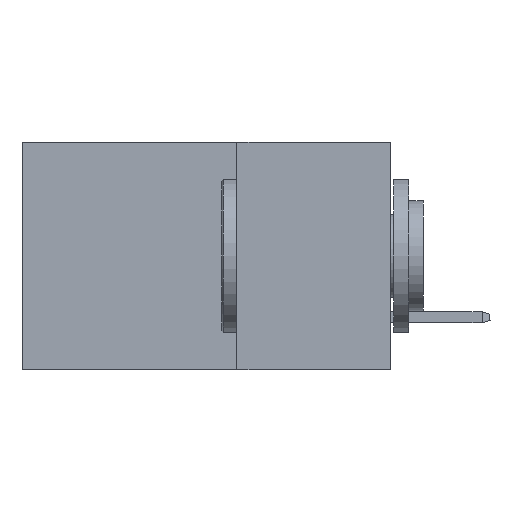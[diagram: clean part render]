
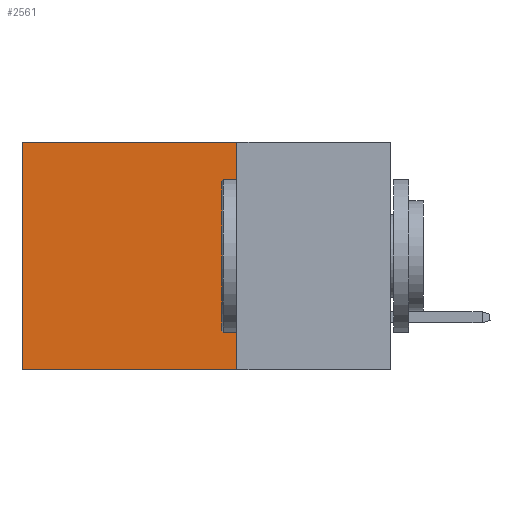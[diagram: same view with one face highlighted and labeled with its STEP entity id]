
A CAD part, left-side view. The second image highlights one B-rep face of the part: STEP entity #2561.
In plain terms, the highlighted planar face has unit normal (-1, 0, 0).
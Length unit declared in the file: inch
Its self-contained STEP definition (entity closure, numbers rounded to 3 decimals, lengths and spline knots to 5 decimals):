
#837 = CARTESIAN_POINT ( 'NONE',  ( 0.2875, 0.6, -0.37 ) ) ;
#1887 = LINE ( 'NONE', #3237, #12881 ) ;
#2063 = DIRECTION ( 'NONE',  ( 0., 0., -1. ) ) ;
#2218 = FACE_OUTER_BOUND ( 'NONE', #13181, .T. ) ;
#2438 = VERTEX_POINT ( 'NONE', #11773 ) ;
#2561 = ADVANCED_FACE ( 'NONE', ( #2218 ), #13534, .F. ) ;
#2634 = DIRECTION ( 'NONE',  ( 0., 1., 0. ) ) ;
#2800 = DIRECTION ( 'NONE',  ( 0., 1., 0. ) ) ;
#3237 = CARTESIAN_POINT ( 'NONE',  ( 0.2875, 0.25, 0. ) ) ;
#3707 = CARTESIAN_POINT ( 'NONE',  ( 0.2875, 0.25, -0.37 ) ) ;
#3726 = VECTOR ( 'NONE', #2800, 39.37008 ) ;
#3898 = CARTESIAN_POINT ( 'NONE',  ( 0.2875, 0.25, 0. ) ) ;
#3946 = CARTESIAN_POINT ( 'NONE',  ( 0.2875, 0.25, 0. ) ) ;
#4036 = VERTEX_POINT ( 'NONE', #3707 ) ;
#4352 = CARTESIAN_POINT ( 'NONE',  ( 0.2875, 0.25, 0. ) ) ;
#4576 = CARTESIAN_POINT ( 'NONE',  ( 0.2875, 0.25, -0.37 ) ) ;
#5159 = CARTESIAN_POINT ( 'NONE',  ( 0.2875, 0.6, 0. ) ) ;
#5219 = EDGE_CURVE ( 'NONE', #4036, #9318, #9870, .T. ) ;
#5222 = DIRECTION ( 'NONE',  ( 0., 0., -1. ) ) ;
#5490 = ORIENTED_EDGE ( 'NONE', *, *, #6784, .T. ) ;
#5529 = LINE ( 'NONE', #3946, #3726 ) ;
#5677 = ORIENTED_EDGE ( 'NONE', *, *, #9468, .T. ) ;
#6610 = VECTOR ( 'NONE', #2063, 39.37008 ) ;
#6657 = ORIENTED_EDGE ( 'NONE', *, *, #5219, .F. ) ;
#6784 = EDGE_CURVE ( 'NONE', #2438, #9318, #9489, .T. ) ;
#6973 = DIRECTION ( 'NONE',  ( 1., 0., 0. ) ) ;
#8467 = AXIS2_PLACEMENT_3D ( 'NONE', #3898, #6973, #10251 ) ;
#9035 = ORIENTED_EDGE ( 'NONE', *, *, #10538, .F. ) ;
#9042 = VERTEX_POINT ( 'NONE', #4352 ) ;
#9318 = VERTEX_POINT ( 'NONE', #837 ) ;
#9468 = EDGE_CURVE ( 'NONE', #9042, #2438, #5529, .T. ) ;
#9489 = LINE ( 'NONE', #5159, #6610 ) ;
#9870 = LINE ( 'NONE', #4576, #13000 ) ;
#10251 = DIRECTION ( 'NONE',  ( 0., 0., -1. ) ) ;
#10538 = EDGE_CURVE ( 'NONE', #9042, #4036, #1887, .T. ) ;
#11773 = CARTESIAN_POINT ( 'NONE',  ( 0.2875, 0.6, 0. ) ) ;
#12881 = VECTOR ( 'NONE', #5222, 39.37008 ) ;
#13000 = VECTOR ( 'NONE', #2634, 39.37008 ) ;
#13181 = EDGE_LOOP ( 'NONE', ( #5490, #6657, #9035, #5677 ) ) ;
#13534 = PLANE ( 'NONE',  #8467 ) ;
